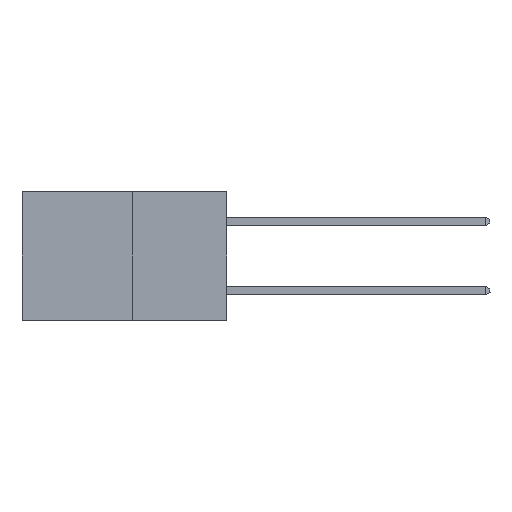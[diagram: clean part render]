
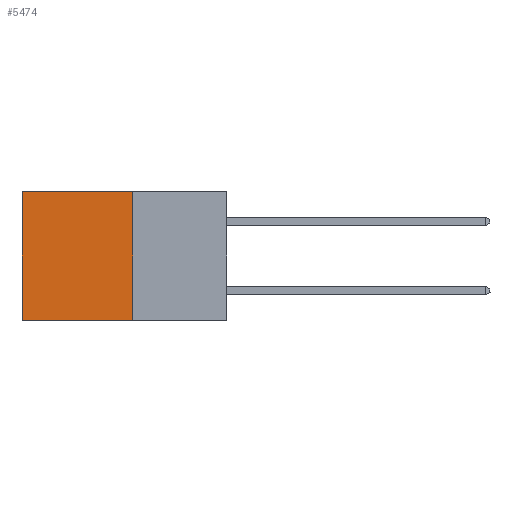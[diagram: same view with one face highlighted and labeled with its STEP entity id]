
A CAD part, left-side view. The second image highlights one B-rep face of the part: STEP entity #5474.
In plain terms, the highlighted planar face has unit normal (-1, 0, 0).
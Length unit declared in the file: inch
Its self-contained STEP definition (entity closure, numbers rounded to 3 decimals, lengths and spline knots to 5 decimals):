
#832 = CARTESIAN_POINT ( 'NONE',  ( 0.277, 0.27, -0.37 ) ) ;
#1282 = VECTOR ( 'NONE', #5600, 39.37008 ) ;
#1434 = DIRECTION ( 'NONE',  ( 0., 0., -1. ) ) ;
#1500 = ORIENTED_EDGE ( 'NONE', *, *, #7981, .T. ) ;
#1655 = CARTESIAN_POINT ( 'NONE',  ( 0.277, 0.27, -0.37 ) ) ;
#2175 = VERTEX_POINT ( 'NONE', #8039 ) ;
#2763 = VERTEX_POINT ( 'NONE', #832 ) ;
#2973 = VERTEX_POINT ( 'NONE', #7681 ) ;
#3077 = EDGE_CURVE ( 'NONE', #2763, #2973, #9223, .T. ) ;
#3548 = VERTEX_POINT ( 'NONE', #7227 ) ;
#3907 = EDGE_LOOP ( 'NONE', ( #1500, #3922, #6068, #7990 ) ) ;
#3922 = ORIENTED_EDGE ( 'NONE', *, *, #3077, .F. ) ;
#4961 = DIRECTION ( 'NONE',  ( 0., 0., -1. ) ) ;
#4964 = DIRECTION ( 'NONE',  ( 1., 0., 0. ) ) ;
#4984 = PLANE ( 'NONE',  #8719 ) ;
#5010 = CARTESIAN_POINT ( 'NONE',  ( 0.277, 0.27, -0.37 ) ) ;
#5301 = VECTOR ( 'NONE', #6442, 39.37008 ) ;
#5474 = ADVANCED_FACE ( 'NONE', ( #10145 ), #4984, .F. ) ;
#5600 = DIRECTION ( 'NONE',  ( 0., 1., 0. ) ) ;
#5815 = CARTESIAN_POINT ( 'NONE',  ( 0.277, 0.27, 0. ) ) ;
#6068 = ORIENTED_EDGE ( 'NONE', *, *, #6719, .F. ) ;
#6124 = VECTOR ( 'NONE', #8941, 39.37008 ) ;
#6439 = CARTESIAN_POINT ( 'NONE',  ( 0.277, 0.27, -0.37 ) ) ;
#6442 = DIRECTION ( 'NONE',  ( 0., 1., 0. ) ) ;
#6490 = LINE ( 'NONE', #1655, #8397 ) ;
#6719 = EDGE_CURVE ( 'NONE', #3548, #2763, #6490, .T. ) ;
#7190 = EDGE_CURVE ( 'NONE', #3548, #2175, #8055, .T. ) ;
#7227 = CARTESIAN_POINT ( 'NONE',  ( 0.277, 0.27, 0. ) ) ;
#7470 = CARTESIAN_POINT ( 'NONE',  ( 0.277, 0.59, -0.37 ) ) ;
#7681 = CARTESIAN_POINT ( 'NONE',  ( 0.277, 0.59, -0.37 ) ) ;
#7981 = EDGE_CURVE ( 'NONE', #2175, #2973, #8493, .T. ) ;
#7990 = ORIENTED_EDGE ( 'NONE', *, *, #7190, .T. ) ;
#8039 = CARTESIAN_POINT ( 'NONE',  ( 0.277, 0.59, 0. ) ) ;
#8055 = LINE ( 'NONE', #5815, #1282 ) ;
#8397 = VECTOR ( 'NONE', #1434, 39.37008 ) ;
#8493 = LINE ( 'NONE', #7470, #6124 ) ;
#8719 = AXIS2_PLACEMENT_3D ( 'NONE', #5010, #4964, #4961 ) ;
#8941 = DIRECTION ( 'NONE',  ( 0., 0., -1. ) ) ;
#9223 = LINE ( 'NONE', #6439, #5301 ) ;
#10145 = FACE_OUTER_BOUND ( 'NONE', #3907, .T. ) ;
